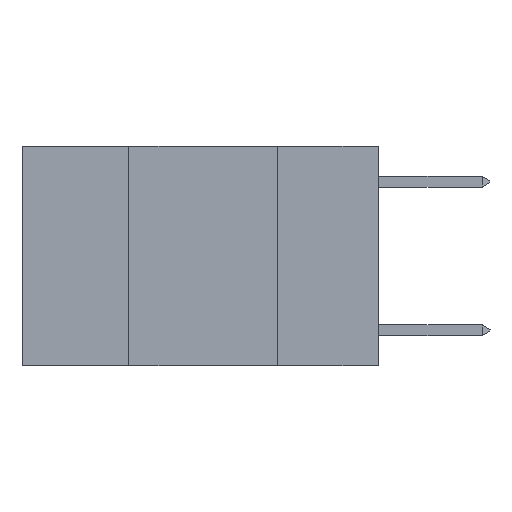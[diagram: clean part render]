
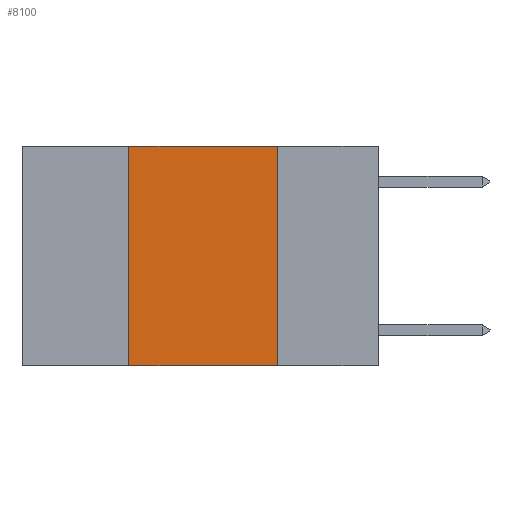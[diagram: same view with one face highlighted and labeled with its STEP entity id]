
A CAD part, left-side view. The second image highlights one B-rep face of the part: STEP entity #8100.
In plain terms, the highlighted planar face has unit normal (-1, 0, 0).
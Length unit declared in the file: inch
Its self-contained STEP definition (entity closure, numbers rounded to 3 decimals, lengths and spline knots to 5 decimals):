
#2577 = VERTEX_POINT ( 'NONE', #4327 ) ;
#3101 = EDGE_CURVE ( 'NONE', #9241, #9992, #7909, .T. ) ;
#3456 = CARTESIAN_POINT ( 'NONE',  ( 0., 0.42, 0. ) ) ;
#3642 = ORIENTED_EDGE ( 'NONE', *, *, #21542, .T. ) ;
#4327 = CARTESIAN_POINT ( 'NONE',  ( 0., 0.42, -0.37 ) ) ;
#4590 = EDGE_LOOP ( 'NONE', ( #19657, #9995, #13318, #3642 ) ) ;
#5750 = DIRECTION ( 'NONE',  ( 0., 0., -1. ) ) ;
#7019 = DIRECTION ( 'NONE',  ( 0., 0., -1. ) ) ;
#7048 = DIRECTION ( 'NONE',  ( 1., 0., 0. ) ) ;
#7123 = PLANE ( 'NONE',  #22993 ) ;
#7148 = CARTESIAN_POINT ( 'NONE',  ( 0., 0.6, 0. ) ) ;
#7379 = VECTOR ( 'NONE', #10121, 39.37008 ) ;
#7486 = LINE ( 'NONE', #19146, #7379 ) ;
#7840 = VECTOR ( 'NONE', #22389, 39.37008 ) ;
#7909 = LINE ( 'NONE', #22410, #7840 ) ;
#8100 = ADVANCED_FACE ( 'NONE', ( #9486 ), #7123, .F. ) ;
#9241 = VERTEX_POINT ( 'NONE', #19796 ) ;
#9315 = VERTEX_POINT ( 'NONE', #17905 ) ;
#9412 = CARTESIAN_POINT ( 'NONE',  ( 0., 0.17, 0. ) ) ;
#9486 = FACE_OUTER_BOUND ( 'NONE', #4590, .T. ) ;
#9992 = VERTEX_POINT ( 'NONE', #19445 ) ;
#9995 = ORIENTED_EDGE ( 'NONE', *, *, #3101, .F. ) ;
#10121 = DIRECTION ( 'NONE',  ( 0., -1., 0. ) ) ;
#11373 = VECTOR ( 'NONE', #14670, 39.37008 ) ;
#11624 = LINE ( 'NONE', #3456, #11373 ) ;
#13318 = ORIENTED_EDGE ( 'NONE', *, *, #18026, .F. ) ;
#14670 = DIRECTION ( 'NONE',  ( 0., 0., 1. ) ) ;
#16927 = EDGE_CURVE ( 'NONE', #9992, #9315, #21242, .T. ) ;
#17905 = CARTESIAN_POINT ( 'NONE',  ( 0., 0.17, -0.37 ) ) ;
#18026 = EDGE_CURVE ( 'NONE', #2577, #9241, #11624, .T. ) ;
#19146 = CARTESIAN_POINT ( 'NONE',  ( 0., 0.6, -0.37 ) ) ;
#19445 = CARTESIAN_POINT ( 'NONE',  ( 0., 0.17, 0. ) ) ;
#19657 = ORIENTED_EDGE ( 'NONE', *, *, #16927, .F. ) ;
#19796 = CARTESIAN_POINT ( 'NONE',  ( 0., 0.42, 0. ) ) ;
#20668 = VECTOR ( 'NONE', #5750, 39.37008 ) ;
#21242 = LINE ( 'NONE', #9412, #20668 ) ;
#21542 = EDGE_CURVE ( 'NONE', #2577, #9315, #7486, .T. ) ;
#22389 = DIRECTION ( 'NONE',  ( 0., -1., 0. ) ) ;
#22410 = CARTESIAN_POINT ( 'NONE',  ( 0., 0.6, 0. ) ) ;
#22993 = AXIS2_PLACEMENT_3D ( 'NONE', #7148, #7048, #7019 ) ;
